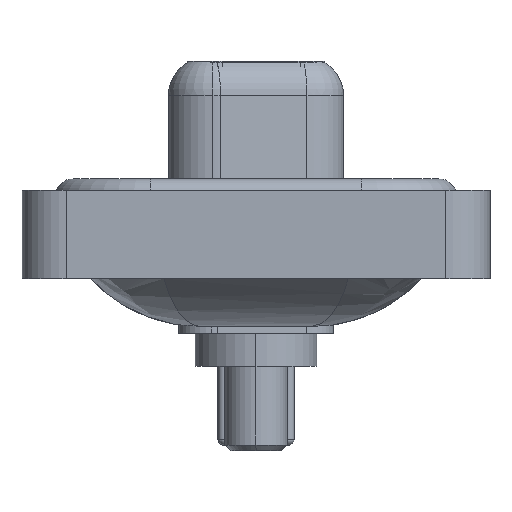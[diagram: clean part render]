
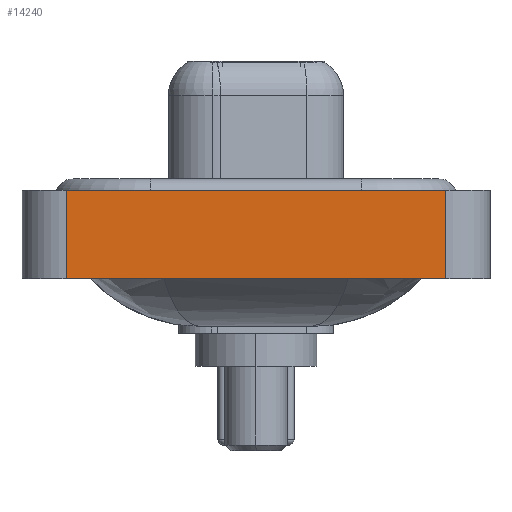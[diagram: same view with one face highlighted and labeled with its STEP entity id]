
A CAD part, left-side view. The second image highlights one B-rep face of the part: STEP entity #14240.
In plain terms, the highlighted planar face has unit normal (-1, 0, 0).
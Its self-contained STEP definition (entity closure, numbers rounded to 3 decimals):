
#906 = VERTEX_POINT ( 'NONE', #1708 ) ;
#1042 = VECTOR ( 'NONE', #4565, 1000. ) ;
#1708 = CARTESIAN_POINT ( 'NONE',  ( -7.35, 8.55, 0.4 ) ) ;
#1937 = EDGE_CURVE ( 'NONE', #11338, #10807, #16636, .T. ) ;
#2336 = EDGE_CURVE ( 'NONE', #11338, #906, #8299, .T. ) ;
#2575 = CARTESIAN_POINT ( 'NONE',  ( -7.35, 8.55, -3.6 ) ) ;
#3091 = ORIENTED_EDGE ( 'NONE', *, *, #2336, .F. ) ;
#3152 = CARTESIAN_POINT ( 'NONE',  ( -7.35, -8.55, -3.6 ) ) ;
#3562 = CARTESIAN_POINT ( 'NONE',  ( -7.35, -8.55, 0.4 ) ) ;
#3934 = CARTESIAN_POINT ( 'NONE',  ( -7.35, -8.55, 0.4 ) ) ;
#3961 = EDGE_LOOP ( 'NONE', ( #12881, #22500, #3091, #13914 ) ) ;
#3977 = EDGE_CURVE ( 'NONE', #10807, #17157, #22584, .T. ) ;
#4565 = DIRECTION ( 'NONE',  ( 0., 0., 1. ) ) ;
#6448 = VECTOR ( 'NONE', #18735, 1000. ) ;
#8299 = LINE ( 'NONE', #2575, #1042 ) ;
#10179 = DIRECTION ( 'NONE',  ( -1., 0., 0. ) ) ;
#10656 = FACE_OUTER_BOUND ( 'NONE', #3961, .T. ) ;
#10807 = VERTEX_POINT ( 'NONE', #3152 ) ;
#11338 = VERTEX_POINT ( 'NONE', #22524 ) ;
#12150 = DIRECTION ( 'NONE',  ( 0., 0., 1. ) ) ;
#12777 = DIRECTION ( 'NONE',  ( 0., -1., 0. ) ) ;
#12881 = ORIENTED_EDGE ( 'NONE', *, *, #3977, .T. ) ;
#13251 = CARTESIAN_POINT ( 'NONE',  ( -7.35, -8.55, -3.6 ) ) ;
#13914 = ORIENTED_EDGE ( 'NONE', *, *, #1937, .T. ) ;
#14021 = PLANE ( 'NONE',  #22191 ) ;
#14240 = ADVANCED_FACE ( 'NONE', ( #10656 ), #14021, .T. ) ;
#14774 = CARTESIAN_POINT ( 'NONE',  ( -7.35, -8.55, -3.6 ) ) ;
#16636 = LINE ( 'NONE', #14774, #19861 ) ;
#16998 = EDGE_CURVE ( 'NONE', #906, #17157, #17003, .T. ) ;
#17003 = LINE ( 'NONE', #3562, #6448 ) ;
#17157 = VERTEX_POINT ( 'NONE', #3934 ) ;
#18735 = DIRECTION ( 'NONE',  ( 0., -1., 0. ) ) ;
#19861 = VECTOR ( 'NONE', #12777, 1000. ) ;
#22191 = AXIS2_PLACEMENT_3D ( 'NONE', #23709, #10179, #12150 ) ;
#22500 = ORIENTED_EDGE ( 'NONE', *, *, #16998, .F. ) ;
#22524 = CARTESIAN_POINT ( 'NONE',  ( -7.35, 8.55, -3.6 ) ) ;
#22584 = LINE ( 'NONE', #13251, #24145 ) ;
#23709 = CARTESIAN_POINT ( 'NONE',  ( -7.35, -8.55, -3.6 ) ) ;
#24145 = VECTOR ( 'NONE', #24448, 1000. ) ;
#24448 = DIRECTION ( 'NONE',  ( 0., 0., 1. ) ) ;
